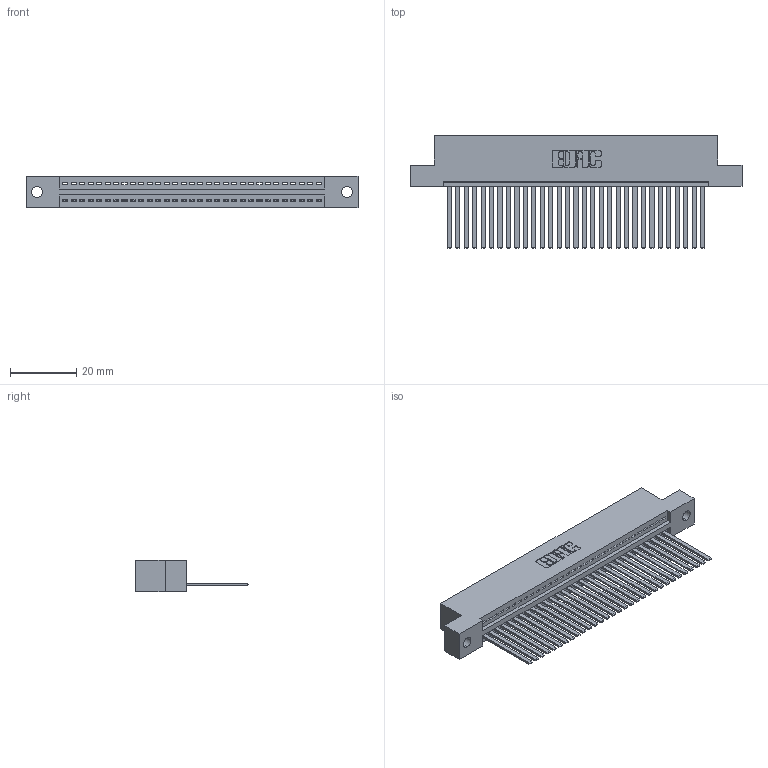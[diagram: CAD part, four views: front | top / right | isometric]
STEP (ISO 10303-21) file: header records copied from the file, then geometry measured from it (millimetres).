
FILE_DESCRIPTION (( 'STEP AP203' ), '1' );
FILE_NAME ('345-031-544-102.STEP', '2019-10-07T13:00:16', ( '' ), ( '' ), 'SwSTEP 2.0', 'SolidWorks 2016', '' );
FILE_SCHEMA (( 'CONFIG_CONTROL_DESIGN' ));
Length unit declared in the file: inch
Products named in the file (3): 345-292-001_345-293-144; 345-031-544-102; 345 Part_Flush Mounting Lugs - 0.128 Dia
Assembly tree (32 placements, depth 2):
  345-031-544-102
    345 Part_Flush Mounting Lugs - 0.128 Dia
    345-292-001_345-293-144  x31
Bounding box: 99.95 x 33.96 x 9.4 mm (x, y, z)
Volume: 9725.5 mm3; surface area: 13581.1 mm2
Topology: 32 solids, 32 shells, 1738 faces, 5239 edges, 3450 vertices
Faces by surface type: plane 1196, cylinder 542
Entity records: 24631 total; most frequent: CARTESIAN_POINT 4273, ORIENTED_EDGE 4238, DIRECTION 3745, EDGE_CURVE 2119, LINE 1867, VECTOR 1867, VERTEX_POINT 1410, AXIS2_PLACEMENT_3D 939
